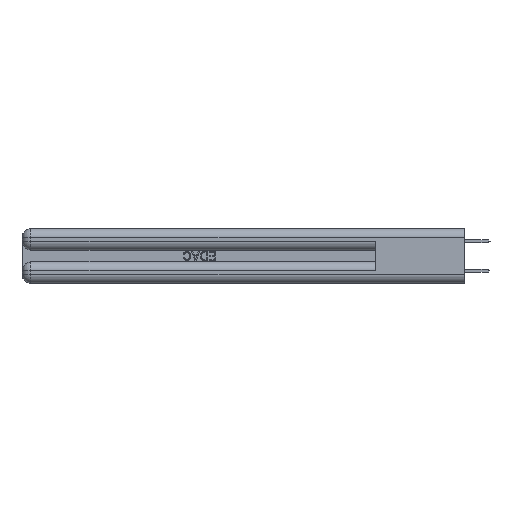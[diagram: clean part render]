
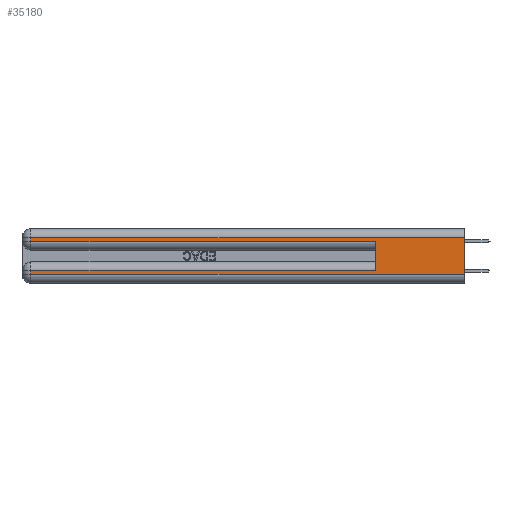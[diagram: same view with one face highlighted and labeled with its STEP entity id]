
A CAD part, left-side view. The second image highlights one B-rep face of the part: STEP entity #35180.
In plain terms, the highlighted planar face has unit normal (-1, 0, 0).
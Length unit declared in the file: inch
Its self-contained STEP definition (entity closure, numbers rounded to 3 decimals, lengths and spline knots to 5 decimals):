
#636 = VECTOR ( 'NONE', #13673, 39.37008 ) ;
#915 = DIRECTION ( 'NONE',  ( 1., 0., 0. ) ) ;
#1667 = LINE ( 'NONE', #26536, #636 ) ;
#1758 = CARTESIAN_POINT ( 'NONE',  ( 0., 0.6, 0.085 ) ) ;
#2311 = VECTOR ( 'NONE', #8525, 39.37008 ) ;
#3395 = VERTEX_POINT ( 'NONE', #23550 ) ;
#3421 = LINE ( 'NONE', #26793, #18443 ) ;
#5301 = CARTESIAN_POINT ( 'NONE',  ( 0., 0.6, 0.145 ) ) ;
#5415 = LINE ( 'NONE', #37473, #29931 ) ;
#5452 = FACE_OUTER_BOUND ( 'NONE', #31208, .T. ) ;
#5467 = VERTEX_POINT ( 'NONE', #6400 ) ;
#5968 = CARTESIAN_POINT ( 'NONE',  ( 0., 0., 0.06 ) ) ;
#6400 = CARTESIAN_POINT ( 'NONE',  ( 0., 2.94, 0.285 ) ) ;
#6504 = VERTEX_POINT ( 'NONE', #13730 ) ;
#6952 = VERTEX_POINT ( 'NONE', #34989 ) ;
#7262 = LINE ( 'NONE', #7459, #40398 ) ;
#7459 = CARTESIAN_POINT ( 'NONE',  ( 0., 2.94, 0.37 ) ) ;
#7897 = VERTEX_POINT ( 'NONE', #1758 ) ;
#8525 = DIRECTION ( 'NONE',  ( 0., 0., 1. ) ) ;
#9204 = DIRECTION ( 'NONE',  ( 0., -1., 0. ) ) ;
#9674 = EDGE_CURVE ( 'NONE', #19275, #6504, #30219, .T. ) ;
#9912 = DIRECTION ( 'NONE',  ( 0., 0., -1. ) ) ;
#10429 = PLANE ( 'NONE',  #33011 ) ;
#12619 = ORIENTED_EDGE ( 'NONE', *, *, #35271, .T. ) ;
#13487 = ORIENTED_EDGE ( 'NONE', *, *, #18342, .T. ) ;
#13673 = DIRECTION ( 'NONE',  ( 0., 1., 0. ) ) ;
#13730 = CARTESIAN_POINT ( 'NONE',  ( 0., 0., 0.06 ) ) ;
#14204 = VECTOR ( 'NONE', #26266, 39.37008 ) ;
#16564 = CARTESIAN_POINT ( 'NONE',  ( 0., 2.94, 0.31 ) ) ;
#16683 = DIRECTION ( 'NONE',  ( 0., 0., -1. ) ) ;
#18342 = EDGE_CURVE ( 'NONE', #19275, #27688, #1667, .T. ) ;
#18443 = VECTOR ( 'NONE', #30152, 39.37008 ) ;
#19275 = VERTEX_POINT ( 'NONE', #28160 ) ;
#20053 = CARTESIAN_POINT ( 'NONE',  ( 0., 0., 0.37 ) ) ;
#22138 = LINE ( 'NONE', #5968, #38256 ) ;
#22446 = EDGE_CURVE ( 'NONE', #27688, #5467, #7262, .T. ) ;
#22698 = VECTOR ( 'NONE', #9912, 39.37008 ) ;
#23039 = CARTESIAN_POINT ( 'NONE',  ( 0., 0., 0.285 ) ) ;
#23289 = DIRECTION ( 'NONE',  ( 0., 0., -1. ) ) ;
#23550 = CARTESIAN_POINT ( 'NONE',  ( 0., 0.6, 0.285 ) ) ;
#23727 = LINE ( 'NONE', #23039, #14204 ) ;
#23880 = EDGE_CURVE ( 'NONE', #5467, #3395, #23727, .T. ) ;
#26266 = DIRECTION ( 'NONE',  ( 0., -1., 0. ) ) ;
#26536 = CARTESIAN_POINT ( 'NONE',  ( 0., 0., 0.31 ) ) ;
#26728 = CARTESIAN_POINT ( 'NONE',  ( 0., 2.94, 0.06 ) ) ;
#26793 = CARTESIAN_POINT ( 'NONE',  ( 0., 0., 0.085 ) ) ;
#27688 = VERTEX_POINT ( 'NONE', #16564 ) ;
#27829 = LINE ( 'NONE', #5301, #2311 ) ;
#28160 = CARTESIAN_POINT ( 'NONE',  ( 0., 0., 0.31 ) ) ;
#28508 = VERTEX_POINT ( 'NONE', #26728 ) ;
#29054 = CARTESIAN_POINT ( 'NONE',  ( 0., 0., 0.37 ) ) ;
#29551 = EDGE_CURVE ( 'NONE', #7897, #3395, #27829, .T. ) ;
#29931 = VECTOR ( 'NONE', #16683, 39.37008 ) ;
#30152 = DIRECTION ( 'NONE',  ( 0., 1., 0. ) ) ;
#30219 = LINE ( 'NONE', #29054, #22698 ) ;
#31208 = EDGE_LOOP ( 'NONE', ( #37960, #13487, #31340, #41231, #37487, #12619, #35341, #32732 ) ) ;
#31340 = ORIENTED_EDGE ( 'NONE', *, *, #22446, .T. ) ;
#32732 = ORIENTED_EDGE ( 'NONE', *, *, #33087, .T. ) ;
#33011 = AXIS2_PLACEMENT_3D ( 'NONE', #20053, #915, #23289 ) ;
#33087 = EDGE_CURVE ( 'NONE', #28508, #6504, #22138, .T. ) ;
#34989 = CARTESIAN_POINT ( 'NONE',  ( 0., 2.94, 0.085 ) ) ;
#35180 = ADVANCED_FACE ( 'NONE', ( #5452 ), #10429, .F. ) ;
#35271 = EDGE_CURVE ( 'NONE', #7897, #6952, #3421, .T. ) ;
#35341 = ORIENTED_EDGE ( 'NONE', *, *, #35403, .T. ) ;
#35403 = EDGE_CURVE ( 'NONE', #6952, #28508, #5415, .T. ) ;
#36299 = DIRECTION ( 'NONE',  ( 0., 0., -1. ) ) ;
#37473 = CARTESIAN_POINT ( 'NONE',  ( 0., 2.94, 0.37 ) ) ;
#37487 = ORIENTED_EDGE ( 'NONE', *, *, #29551, .F. ) ;
#37960 = ORIENTED_EDGE ( 'NONE', *, *, #9674, .F. ) ;
#38256 = VECTOR ( 'NONE', #9204, 39.37008 ) ;
#40398 = VECTOR ( 'NONE', #36299, 39.37008 ) ;
#41231 = ORIENTED_EDGE ( 'NONE', *, *, #23880, .T. ) ;
